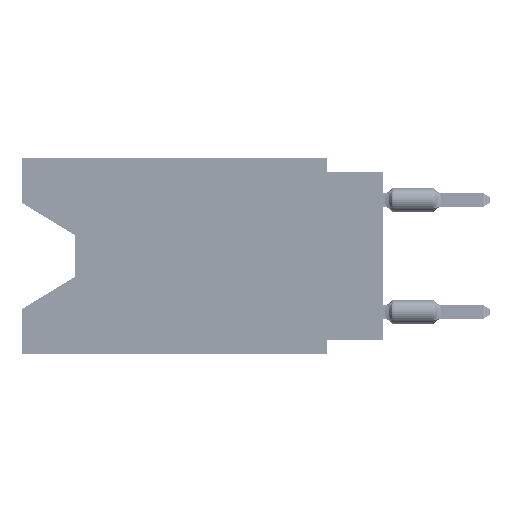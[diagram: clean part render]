
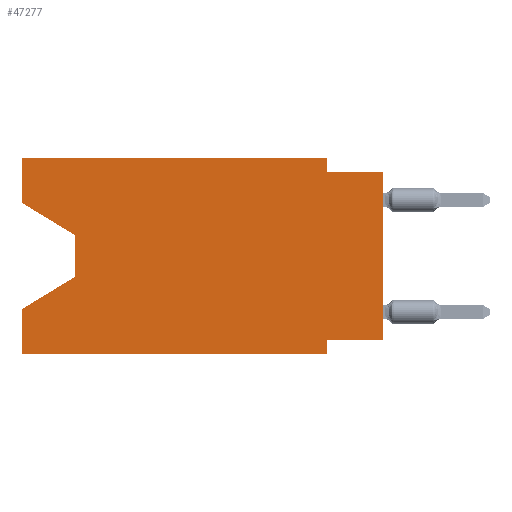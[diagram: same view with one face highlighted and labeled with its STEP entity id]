
A CAD part, left-side view. The second image highlights one B-rep face of the part: STEP entity #47277.
In plain terms, the highlighted planar face has unit normal (-1, 0, 0).
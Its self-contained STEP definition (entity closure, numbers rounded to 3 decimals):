
#1218 = VECTOR ( 'NONE', #14651, 1000. ) ;
#3564 = ORIENTED_EDGE ( 'NONE', *, *, #74790, .F. ) ;
#4069 = VERTEX_POINT ( 'NONE', #7348 ) ;
#4156 = DIRECTION ( 'NONE',  ( 0., 0., -1. ) ) ;
#6496 = EDGE_CURVE ( 'NONE', #25710, #89973, #40417, .T. ) ;
#6616 = CARTESIAN_POINT ( 'NONE',  ( 0., 13.97, -5.385 ) ) ;
#7348 = CARTESIAN_POINT ( 'NONE',  ( 0., 2.54, -0.635 ) ) ;
#10493 = LINE ( 'NONE', #61492, #92535 ) ;
#13365 = ORIENTED_EDGE ( 'NONE', *, *, #36616, .F. ) ;
#14651 = DIRECTION ( 'NONE',  ( 0., 0., 1. ) ) ;
#15078 = DIRECTION ( 'NONE',  ( 0., 0., -1. ) ) ;
#16018 = CARTESIAN_POINT ( 'NONE',  ( 0., 16.383, -2.038 ) ) ;
#19591 = CARTESIAN_POINT ( 'NONE',  ( 0., 2.54, 0. ) ) ;
#23131 = EDGE_CURVE ( 'NONE', #51698, #58708, #10493, .T. ) ;
#23406 = VECTOR ( 'NONE', #4156, 1000. ) ;
#23753 = EDGE_CURVE ( 'NONE', #66924, #89973, #79764, .T. ) ;
#24005 = EDGE_LOOP ( 'NONE', ( #29609, #45088, #55312, #65773, #85485, #81107, #25937, #73427, #3564, #13365, #81867, #33985 ) ) ;
#24206 = DIRECTION ( 'NONE',  ( 0., 0., 1. ) ) ;
#24847 = EDGE_CURVE ( 'NONE', #63870, #25710, #27648, .T. ) ;
#25517 = VERTEX_POINT ( 'NONE', #73174 ) ;
#25643 = VECTOR ( 'NONE', #64060, 1000. ) ;
#25710 = VERTEX_POINT ( 'NONE', #75079 ) ;
#25937 = ORIENTED_EDGE ( 'NONE', *, *, #24847, .F. ) ;
#26722 = CARTESIAN_POINT ( 'NONE',  ( 0., 0., -8.255 ) ) ;
#26936 = CARTESIAN_POINT ( 'NONE',  ( 0., 2.54, 0. ) ) ;
#27610 = DIRECTION ( 'NONE',  ( 0., 0.855, -0.519 ) ) ;
#27648 = LINE ( 'NONE', #26722, #58544 ) ;
#29609 = ORIENTED_EDGE ( 'NONE', *, *, #83911, .T. ) ;
#32201 = VECTOR ( 'NONE', #47268, 1000. ) ;
#32678 = CARTESIAN_POINT ( 'NONE',  ( 0., 16.383, 0. ) ) ;
#33895 = LINE ( 'NONE', #19591, #78219 ) ;
#33985 = ORIENTED_EDGE ( 'NONE', *, *, #80933, .F. ) ;
#35168 = VECTOR ( 'NONE', #87226, 1000. ) ;
#35177 = CARTESIAN_POINT ( 'NONE',  ( 0., 16.383, 0. ) ) ;
#36373 = CARTESIAN_POINT ( 'NONE',  ( 0., 16.383, -8.89 ) ) ;
#36616 = EDGE_CURVE ( 'NONE', #58708, #4069, #33895, .T. ) ;
#40417 = LINE ( 'NONE', #69496, #23406 ) ;
#41519 = VERTEX_POINT ( 'NONE', #51474 ) ;
#41524 = DIRECTION ( 'NONE',  ( 0., 0., -1. ) ) ;
#42235 = CARTESIAN_POINT ( 'NONE',  ( 0., 0., -8.255 ) ) ;
#42740 = CARTESIAN_POINT ( 'NONE',  ( 0., 16.383, 0. ) ) ;
#42860 = VERTEX_POINT ( 'NONE', #57630 ) ;
#45088 = ORIENTED_EDGE ( 'NONE', *, *, #61085, .T. ) ;
#46110 = VECTOR ( 'NONE', #27610, 1000. ) ;
#46706 = CARTESIAN_POINT ( 'NONE',  ( 0., 13.97, -3.505 ) ) ;
#47268 = DIRECTION ( 'NONE',  ( 0., -1., 0. ) ) ;
#47277 = ADVANCED_FACE ( 'NONE', ( #78984 ), #65145, .F. ) ;
#49525 = LINE ( 'NONE', #6616, #46110 ) ;
#49963 = EDGE_CURVE ( 'NONE', #58018, #42860, #49525, .T. ) ;
#50768 = VERTEX_POINT ( 'NONE', #46706 ) ;
#51474 = CARTESIAN_POINT ( 'NONE',  ( 0., 16.383, -2.038 ) ) ;
#51698 = VERTEX_POINT ( 'NONE', #82707 ) ;
#55312 = ORIENTED_EDGE ( 'NONE', *, *, #49963, .T. ) ;
#56438 = CARTESIAN_POINT ( 'NONE',  ( 0., 13.97, -5.385 ) ) ;
#57630 = CARTESIAN_POINT ( 'NONE',  ( 0., 16.383, -6.852 ) ) ;
#57669 = LINE ( 'NONE', #79606, #35168 ) ;
#58018 = VERTEX_POINT ( 'NONE', #56438 ) ;
#58544 = VECTOR ( 'NONE', #91552, 1000. ) ;
#58708 = VERTEX_POINT ( 'NONE', #26936 ) ;
#60423 = LINE ( 'NONE', #89519, #76386 ) ;
#61085 = EDGE_CURVE ( 'NONE', #50768, #58018, #57669, .T. ) ;
#61492 = CARTESIAN_POINT ( 'NONE',  ( 0., 16.383, 0. ) ) ;
#61578 = CARTESIAN_POINT ( 'NONE',  ( 0., 0., -0.635 ) ) ;
#62978 = CARTESIAN_POINT ( 'NONE',  ( 0., 2.54, -8.89 ) ) ;
#63870 = VERTEX_POINT ( 'NONE', #42235 ) ;
#64060 = DIRECTION ( 'NONE',  ( 0., -1., 0. ) ) ;
#64934 = CARTESIAN_POINT ( 'NONE',  ( 0., 16.383, -8.89 ) ) ;
#65145 = PLANE ( 'NONE',  #65474 ) ;
#65474 = AXIS2_PLACEMENT_3D ( 'NONE', #42740, #87073, #15078 ) ;
#65773 = ORIENTED_EDGE ( 'NONE', *, *, #69152, .F. ) ;
#65915 = VECTOR ( 'NONE', #69872, 1000. ) ;
#66924 = VERTEX_POINT ( 'NONE', #64934 ) ;
#69152 = EDGE_CURVE ( 'NONE', #66924, #42860, #86184, .T. ) ;
#69496 = CARTESIAN_POINT ( 'NONE',  ( 0., 2.54, -8.89 ) ) ;
#69872 = DIRECTION ( 'NONE',  ( 0., 0., 1. ) ) ;
#73174 = CARTESIAN_POINT ( 'NONE',  ( 0., 0., -0.635 ) ) ;
#73269 = EDGE_CURVE ( 'NONE', #63870, #25517, #60423, .T. ) ;
#73427 = ORIENTED_EDGE ( 'NONE', *, *, #73269, .T. ) ;
#74790 = EDGE_CURVE ( 'NONE', #4069, #25517, #83971, .T. ) ;
#75079 = CARTESIAN_POINT ( 'NONE',  ( 0., 2.54, -8.255 ) ) ;
#76386 = VECTOR ( 'NONE', #24206, 1000. ) ;
#78219 = VECTOR ( 'NONE', #41524, 1000. ) ;
#78984 = FACE_OUTER_BOUND ( 'NONE', #24005, .T. ) ;
#79606 = CARTESIAN_POINT ( 'NONE',  ( 0., 13.97, -3.505 ) ) ;
#79764 = LINE ( 'NONE', #36373, #25643 ) ;
#80933 = EDGE_CURVE ( 'NONE', #41519, #51698, #82761, .T. ) ;
#81107 = ORIENTED_EDGE ( 'NONE', *, *, #6496, .F. ) ;
#81333 = LINE ( 'NONE', #16018, #85905 ) ;
#81867 = ORIENTED_EDGE ( 'NONE', *, *, #23131, .F. ) ;
#82707 = CARTESIAN_POINT ( 'NONE',  ( 0., 16.383, 0. ) ) ;
#82761 = LINE ( 'NONE', #32678, #65915 ) ;
#82973 = DIRECTION ( 'NONE',  ( 0., -1., 0. ) ) ;
#83911 = EDGE_CURVE ( 'NONE', #41519, #50768, #81333, .T. ) ;
#83971 = LINE ( 'NONE', #61578, #32201 ) ;
#85485 = ORIENTED_EDGE ( 'NONE', *, *, #23753, .T. ) ;
#85905 = VECTOR ( 'NONE', #88946, 1000. ) ;
#86184 = LINE ( 'NONE', #35177, #1218 ) ;
#87073 = DIRECTION ( 'NONE',  ( 1., 0., 0. ) ) ;
#87226 = DIRECTION ( 'NONE',  ( 0., 0., -1. ) ) ;
#88946 = DIRECTION ( 'NONE',  ( 0., -0.855, -0.519 ) ) ;
#89519 = CARTESIAN_POINT ( 'NONE',  ( 0., 0., 0. ) ) ;
#89973 = VERTEX_POINT ( 'NONE', #62978 ) ;
#91552 = DIRECTION ( 'NONE',  ( 0., 1., 0. ) ) ;
#92535 = VECTOR ( 'NONE', #82973, 1000. ) ;
